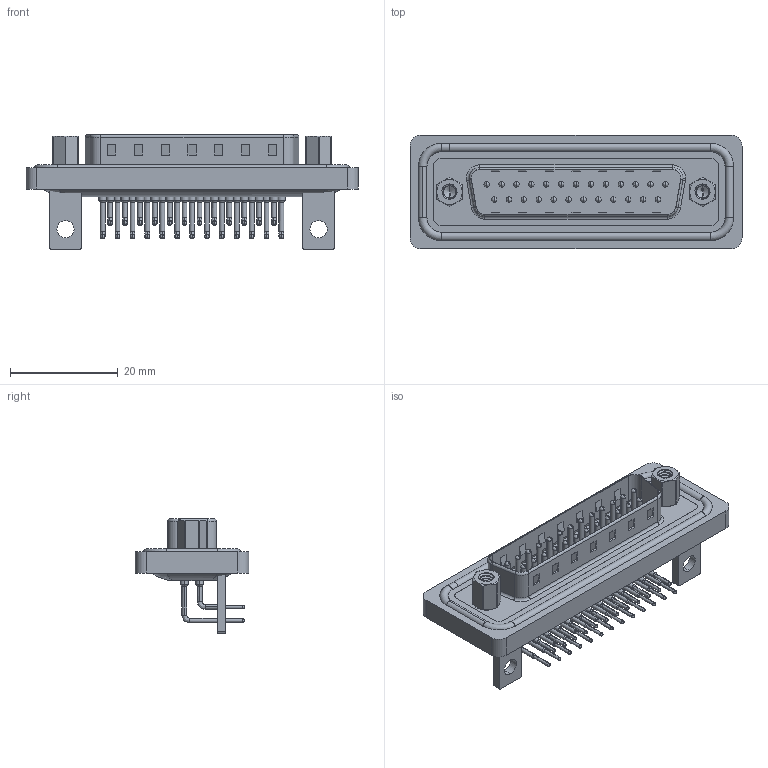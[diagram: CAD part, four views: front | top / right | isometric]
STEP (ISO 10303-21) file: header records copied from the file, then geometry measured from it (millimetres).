
FILE_DESCRIPTION (( 'STEP AP203' ), '1' );
FILE_NAME ('629-W25-240-015.STEP', '2019-08-09T17:44:44', ( '' ), ( '' ), 'SwSTEP 2.0', 'SolidWorks 2016', '' );
FILE_SCHEMA (( 'CONFIG_CONTROL_DESIGN' ));
Length unit declared in the file: millimetre
Products named in the file (9): 629-W25-240-015; 629W Waterproof Housing_25 Contacts; 629W Stabilizer Bracket; 629W Contact Row 2; 629W Housing_25 Contacts; 629W 4-40 Hex Standoff; 629W 4-40 Threaded Rivet_Stabilizer; 629W Contact Row 1; 629W Shell_25 Contacts
Assembly tree (34 placements, depth 2):
  629-W25-240-015
    629W Housing_25 Contacts
    629W Shell_25 Contacts
    629W Waterproof Housing_25 Contacts
    629W Contact Row 1  x13
    629W Contact Row 2  x12
    629W 4-40 Threaded Rivet_Stabilizer  x2
    629W 4-40 Hex Standoff  x2
    629W Stabilizer Bracket  x2
Bounding box: 61.74 x 21.1 x 21.3 mm (x, y, z)
Volume: 6756.1 mm3; surface area: 12139.3 mm2
Topology: 35 solids, 35 shells, 3366 faces, 9396 edges, 6113 vertices
Faces by surface type: plane 1827, cylinder 1190, bspline 172, cone 134, torus 43
Entity records: 33965 total; most frequent: CARTESIAN_POINT 9533, DIRECTION 4907, ORIENTED_EDGE 4650, EDGE_CURVE 2325, AXIS2_PLACEMENT_3D 1809, VERTEX_POINT 1513, LINE 1289, VECTOR 1289
